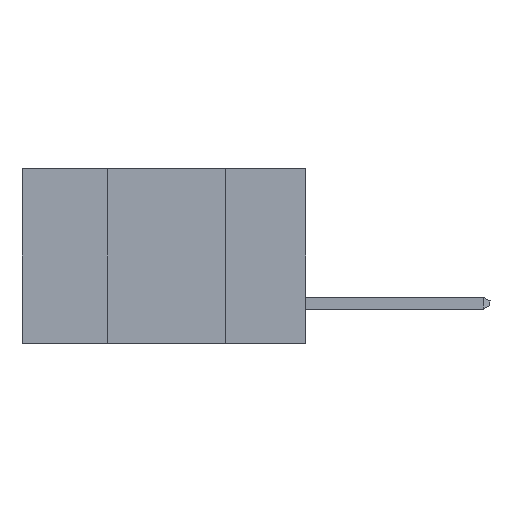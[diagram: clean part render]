
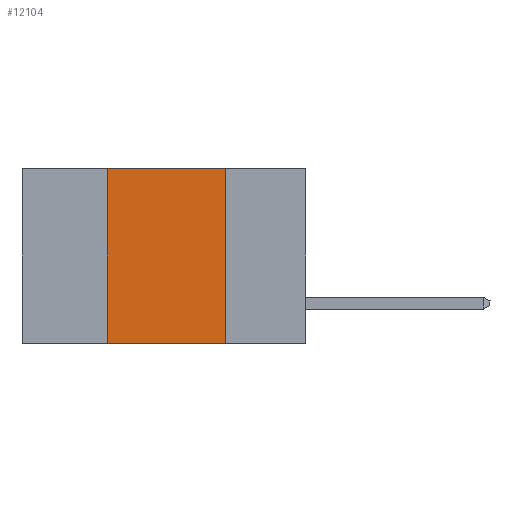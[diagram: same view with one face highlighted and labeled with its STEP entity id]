
A CAD part, left-side view. The second image highlights one B-rep face of the part: STEP entity #12104.
In plain terms, the highlighted planar face has unit normal (-1, 0, 0).
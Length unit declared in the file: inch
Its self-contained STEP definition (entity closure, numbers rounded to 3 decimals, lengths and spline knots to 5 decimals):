
#87 = EDGE_CURVE ( 'NONE', #220, #15295, #12374, .T. ) ;
#220 = VERTEX_POINT ( 'NONE', #12916 ) ;
#341 = VECTOR ( 'NONE', #7588, 39.37008 ) ;
#1907 = LINE ( 'NONE', #4220, #3934 ) ;
#1973 = ORIENTED_EDGE ( 'NONE', *, *, #5726, .F. ) ;
#2032 = CARTESIAN_POINT ( 'NONE',  ( 0., 0.6, 0. ) ) ;
#2065 = DIRECTION ( 'NONE',  ( 0., -1., 0. ) ) ;
#2304 = EDGE_CURVE ( 'NONE', #4017, #8210, #2570, .T. ) ;
#2570 = LINE ( 'NONE', #10249, #8926 ) ;
#2743 = VECTOR ( 'NONE', #11179, 39.37008 ) ;
#3908 = CARTESIAN_POINT ( 'NONE',  ( 0., 0.17, 0. ) ) ;
#3934 = VECTOR ( 'NONE', #2065, 39.37008 ) ;
#4017 = VERTEX_POINT ( 'NONE', #3908 ) ;
#4041 = EDGE_LOOP ( 'NONE', ( #15511, #1973, #13168, #8506 ) ) ;
#4220 = CARTESIAN_POINT ( 'NONE',  ( 0., 0.6, 0. ) ) ;
#4914 = EDGE_CURVE ( 'NONE', #220, #8210, #12654, .T. ) ;
#5726 = EDGE_CURVE ( 'NONE', #15295, #4017, #1907, .T. ) ;
#5888 = CARTESIAN_POINT ( 'NONE',  ( 0., 0.17, -0.37 ) ) ;
#6314 = DIRECTION ( 'NONE',  ( 0., 0., -1. ) ) ;
#6340 = CARTESIAN_POINT ( 'NONE',  ( 0., 0.42, -0.37 ) ) ;
#7588 = DIRECTION ( 'NONE',  ( 0., -1., 0. ) ) ;
#8210 = VERTEX_POINT ( 'NONE', #5888 ) ;
#8242 = DIRECTION ( 'NONE',  ( 0., 0., -1. ) ) ;
#8506 = ORIENTED_EDGE ( 'NONE', *, *, #4914, .T. ) ;
#8926 = VECTOR ( 'NONE', #6314, 39.37008 ) ;
#9104 = FACE_OUTER_BOUND ( 'NONE', #4041, .T. ) ;
#9981 = AXIS2_PLACEMENT_3D ( 'NONE', #2032, #15234, #8242 ) ;
#10249 = CARTESIAN_POINT ( 'NONE',  ( 0., 0.17, -0.37 ) ) ;
#11179 = DIRECTION ( 'NONE',  ( 0., 0., 1. ) ) ;
#11246 = CARTESIAN_POINT ( 'NONE',  ( 0., 0.42, 0. ) ) ;
#12104 = ADVANCED_FACE ( 'NONE', ( #9104 ), #12919, .F. ) ;
#12374 = LINE ( 'NONE', #6340, #2743 ) ;
#12654 = LINE ( 'NONE', #14815, #341 ) ;
#12916 = CARTESIAN_POINT ( 'NONE',  ( 0., 0.42, -0.37 ) ) ;
#12919 = PLANE ( 'NONE',  #9981 ) ;
#13168 = ORIENTED_EDGE ( 'NONE', *, *, #87, .F. ) ;
#14815 = CARTESIAN_POINT ( 'NONE',  ( 0., 0.6, -0.37 ) ) ;
#15234 = DIRECTION ( 'NONE',  ( 1., 0., 0. ) ) ;
#15295 = VERTEX_POINT ( 'NONE', #11246 ) ;
#15511 = ORIENTED_EDGE ( 'NONE', *, *, #2304, .F. ) ;
